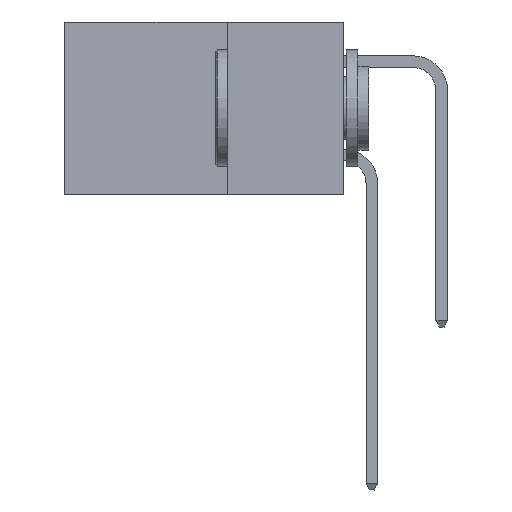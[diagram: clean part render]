
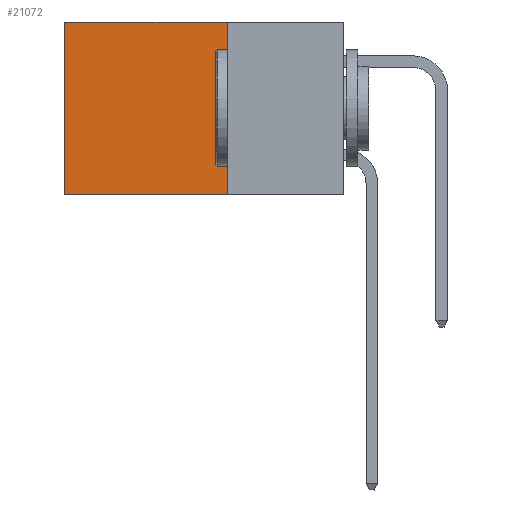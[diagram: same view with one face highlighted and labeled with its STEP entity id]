
A CAD part, left-side view. The second image highlights one B-rep face of the part: STEP entity #21072.
In plain terms, the highlighted planar face has unit normal (-1, 0, 0).
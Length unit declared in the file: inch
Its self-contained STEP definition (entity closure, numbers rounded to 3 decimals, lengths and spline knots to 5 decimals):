
#10 = CARTESIAN_POINT ( 'NONE',  ( 0.298, 0.25, -0.37 ) ) ;
#617 = VERTEX_POINT ( 'NONE', #21042 ) ;
#656 = CARTESIAN_POINT ( 'NONE',  ( 0.298, 0.25, -0.37 ) ) ;
#1167 = VERTEX_POINT ( 'NONE', #13242 ) ;
#1221 = EDGE_CURVE ( 'NONE', #19356, #15071, #4844, .T. ) ;
#1766 = DIRECTION ( 'NONE',  ( 1., 0., 0. ) ) ;
#2490 = LINE ( 'NONE', #24215, #24365 ) ;
#4014 = DIRECTION ( 'NONE',  ( 0., 0., -1. ) ) ;
#4139 = VECTOR ( 'NONE', #15945, 39.37008 ) ;
#4163 = ORIENTED_EDGE ( 'NONE', *, *, #6940, .F. ) ;
#4247 = LINE ( 'NONE', #18282, #16317 ) ;
#4844 = LINE ( 'NONE', #7068, #27781 ) ;
#5023 = EDGE_CURVE ( 'NONE', #1167, #617, #4247, .T. ) ;
#5593 = LINE ( 'NONE', #10, #4139 ) ;
#6123 = PLANE ( 'NONE',  #23116 ) ;
#6940 = EDGE_CURVE ( 'NONE', #15071, #617, #5593, .T. ) ;
#7068 = CARTESIAN_POINT ( 'NONE',  ( 0.298, 0.25, 0. ) ) ;
#9653 = CARTESIAN_POINT ( 'NONE',  ( 0.298, 0.25, 0. ) ) ;
#10175 = FACE_OUTER_BOUND ( 'NONE', #19907, .T. ) ;
#11825 = DIRECTION ( 'NONE',  ( 0., 0., -1. ) ) ;
#13058 = CARTESIAN_POINT ( 'NONE',  ( 0.298, 0.25, 0. ) ) ;
#13242 = CARTESIAN_POINT ( 'NONE',  ( 0.298, 0.6, 0. ) ) ;
#15071 = VERTEX_POINT ( 'NONE', #656 ) ;
#15945 = DIRECTION ( 'NONE',  ( 0., 1., 0. ) ) ;
#16317 = VECTOR ( 'NONE', #22981, 39.37008 ) ;
#18282 = CARTESIAN_POINT ( 'NONE',  ( 0.298, 0.6, 0. ) ) ;
#19173 = ORIENTED_EDGE ( 'NONE', *, *, #5023, .T. ) ;
#19356 = VERTEX_POINT ( 'NONE', #9653 ) ;
#19907 = EDGE_LOOP ( 'NONE', ( #19173, #4163, #25342, #21259 ) ) ;
#21042 = CARTESIAN_POINT ( 'NONE',  ( 0.298, 0.6, -0.37 ) ) ;
#21072 = ADVANCED_FACE ( 'NONE', ( #10175 ), #6123, .F. ) ;
#21259 = ORIENTED_EDGE ( 'NONE', *, *, #25525, .T. ) ;
#22981 = DIRECTION ( 'NONE',  ( 0., 0., -1. ) ) ;
#23116 = AXIS2_PLACEMENT_3D ( 'NONE', #13058, #1766, #4014 ) ;
#24215 = CARTESIAN_POINT ( 'NONE',  ( 0.298, 0.25, 0. ) ) ;
#24365 = VECTOR ( 'NONE', #29009, 39.37008 ) ;
#25342 = ORIENTED_EDGE ( 'NONE', *, *, #1221, .F. ) ;
#25525 = EDGE_CURVE ( 'NONE', #19356, #1167, #2490, .T. ) ;
#27781 = VECTOR ( 'NONE', #11825, 39.37008 ) ;
#29009 = DIRECTION ( 'NONE',  ( 0., 1., 0. ) ) ;
